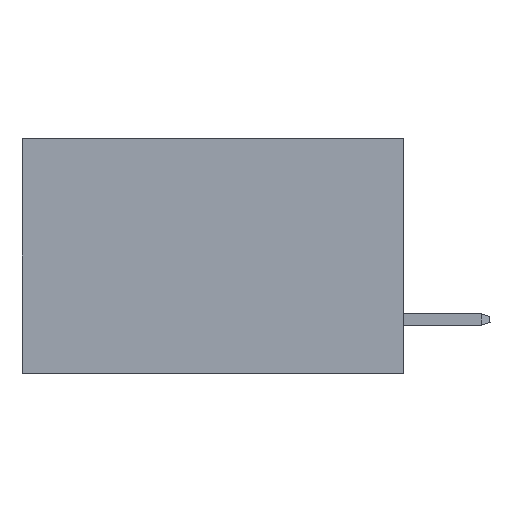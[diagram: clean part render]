
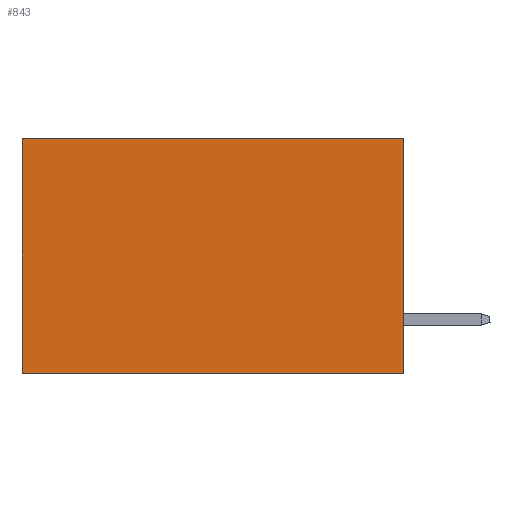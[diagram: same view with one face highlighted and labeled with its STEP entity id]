
A CAD part, left-side view. The second image highlights one B-rep face of the part: STEP entity #843.
In plain terms, the highlighted planar face has unit normal (-1, 0, 0).
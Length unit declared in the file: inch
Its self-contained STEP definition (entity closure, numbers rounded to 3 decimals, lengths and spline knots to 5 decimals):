
#843 = ADVANCED_FACE ( 'NONE', ( #6546 ), #14527, .F. ) ;
#1044 = DIRECTION ( 'NONE',  ( 1., 0., 0. ) ) ;
#1612 = ORIENTED_EDGE ( 'NONE', *, *, #14290, .F. ) ;
#3558 = LINE ( 'NONE', #11561, #8513 ) ;
#3641 = VECTOR ( 'NONE', #4014, 39.37008 ) ;
#4014 = DIRECTION ( 'NONE',  ( 0., 1., 0. ) ) ;
#4155 = CARTESIAN_POINT ( 'NONE',  ( 0.2875, 0., 0. ) ) ;
#6406 = VERTEX_POINT ( 'NONE', #10871 ) ;
#6546 = FACE_OUTER_BOUND ( 'NONE', #9501, .T. ) ;
#8039 = AXIS2_PLACEMENT_3D ( 'NONE', #14903, #1044, #22379 ) ;
#8513 = VECTOR ( 'NONE', #14950, 39.37008 ) ;
#8954 = ORIENTED_EDGE ( 'NONE', *, *, #22866, .F. ) ;
#9501 = EDGE_LOOP ( 'NONE', ( #16476, #8954, #1612, #11029 ) ) ;
#9670 = CARTESIAN_POINT ( 'NONE',  ( 0.2875, 0., -0.37 ) ) ;
#10871 = CARTESIAN_POINT ( 'NONE',  ( 0.2875, 0., -0.37 ) ) ;
#11029 = ORIENTED_EDGE ( 'NONE', *, *, #21640, .T. ) ;
#11500 = CARTESIAN_POINT ( 'NONE',  ( 0.2875, 0., 0. ) ) ;
#11561 = CARTESIAN_POINT ( 'NONE',  ( 0.2875, 0.6, 0. ) ) ;
#11752 = LINE ( 'NONE', #9670, #3641 ) ;
#12139 = VECTOR ( 'NONE', #18145, 39.37008 ) ;
#13437 = VERTEX_POINT ( 'NONE', #21146 ) ;
#13988 = CARTESIAN_POINT ( 'NONE',  ( 0.2875, 0.6, -0.37 ) ) ;
#14290 = EDGE_CURVE ( 'NONE', #22834, #6406, #20238, .T. ) ;
#14527 = PLANE ( 'NONE',  #8039 ) ;
#14691 = CARTESIAN_POINT ( 'NONE',  ( 0.2875, 0., 0. ) ) ;
#14903 = CARTESIAN_POINT ( 'NONE',  ( 0.2875, 0., 0. ) ) ;
#14950 = DIRECTION ( 'NONE',  ( 0., 0., -1. ) ) ;
#16384 = DIRECTION ( 'NONE',  ( 0., 1., 0. ) ) ;
#16476 = ORIENTED_EDGE ( 'NONE', *, *, #18754, .T. ) ;
#18145 = DIRECTION ( 'NONE',  ( 0., 0., -1. ) ) ;
#18478 = LINE ( 'NONE', #14691, #23936 ) ;
#18754 = EDGE_CURVE ( 'NONE', #13437, #20557, #3558, .T. ) ;
#20238 = LINE ( 'NONE', #4155, #12139 ) ;
#20557 = VERTEX_POINT ( 'NONE', #13988 ) ;
#21146 = CARTESIAN_POINT ( 'NONE',  ( 0.2875, 0.6, 0. ) ) ;
#21640 = EDGE_CURVE ( 'NONE', #22834, #13437, #18478, .T. ) ;
#22379 = DIRECTION ( 'NONE',  ( 0., 0., -1. ) ) ;
#22834 = VERTEX_POINT ( 'NONE', #11500 ) ;
#22866 = EDGE_CURVE ( 'NONE', #6406, #20557, #11752, .T. ) ;
#23936 = VECTOR ( 'NONE', #16384, 39.37008 ) ;
